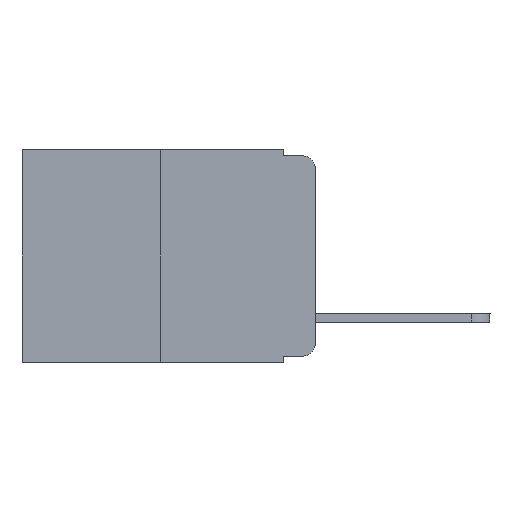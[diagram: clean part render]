
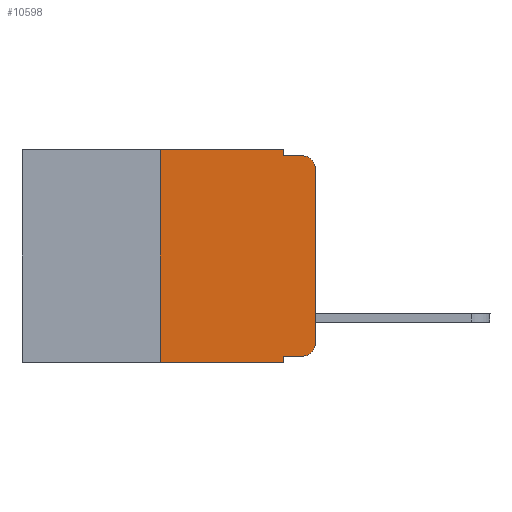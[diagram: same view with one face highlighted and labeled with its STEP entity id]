
A CAD part, left-side view. The second image highlights one B-rep face of the part: STEP entity #10598.
In plain terms, the highlighted planar face has unit normal (-1, 0, 0).
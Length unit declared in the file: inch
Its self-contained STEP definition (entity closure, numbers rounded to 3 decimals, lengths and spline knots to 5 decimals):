
#159 = CARTESIAN_POINT ( 'NONE',  ( 0., 0., -0.03 ) ) ;
#322 = DIRECTION ( 'NONE',  ( 0., 0., 1. ) ) ;
#790 = CARTESIAN_POINT ( 'NONE',  ( 0., 0.473, -0.343 ) ) ;
#799 = ORIENTED_EDGE ( 'NONE', *, *, #14984, .F. ) ;
#1179 = DIRECTION ( 'NONE',  ( 0., 0., -1. ) ) ;
#1741 = VERTEX_POINT ( 'NONE', #6451 ) ;
#1980 = VERTEX_POINT ( 'NONE', #14665 ) ;
#1996 = LINE ( 'NONE', #13366, #11651 ) ;
#2270 = VERTEX_POINT ( 'NONE', #159 ) ;
#2377 = CARTESIAN_POINT ( 'NONE',  ( 0., 0., -0.313 ) ) ;
#2961 = PLANE ( 'NONE',  #17965 ) ;
#2963 = CIRCLE ( 'NONE', #3658, 0.02 ) ;
#3137 = VECTOR ( 'NONE', #13994, 39.37008 ) ;
#3658 = AXIS2_PLACEMENT_3D ( 'NONE', #4294, #9281, #1179 ) ;
#4294 = CARTESIAN_POINT ( 'NONE',  ( 0., 0.02, -0.313 ) ) ;
#4512 = LINE ( 'NONE', #5972, #3137 ) ;
#4913 = LINE ( 'NONE', #14594, #5388 ) ;
#4922 = AXIS2_PLACEMENT_3D ( 'NONE', #5333, #8553, #7001 ) ;
#4974 = ORIENTED_EDGE ( 'NONE', *, *, #9706, .T. ) ;
#5072 = DIRECTION ( 'NONE',  ( 0., -1., 0. ) ) ;
#5231 = DIRECTION ( 'NONE',  ( 0., 0., -1. ) ) ;
#5333 = CARTESIAN_POINT ( 'NONE',  ( 0., 0.02, -0.03 ) ) ;
#5388 = VECTOR ( 'NONE', #322, 39.37008 ) ;
#5605 = VECTOR ( 'NONE', #5231, 39.37008 ) ;
#5791 = DIRECTION ( 'NONE',  ( 1., 0., 0. ) ) ;
#5972 = CARTESIAN_POINT ( 'NONE',  ( 0., 0.051, -0.01 ) ) ;
#6451 = CARTESIAN_POINT ( 'NONE',  ( 0., 0.051, -0.01 ) ) ;
#6452 = VECTOR ( 'NONE', #17511, 39.37008 ) ;
#6668 = EDGE_CURVE ( 'NONE', #1741, #20434, #4512, .T. ) ;
#6861 = ORIENTED_EDGE ( 'NONE', *, *, #16274, .F. ) ;
#6928 = ORIENTED_EDGE ( 'NONE', *, *, #17504, .T. ) ;
#7001 = DIRECTION ( 'NONE',  ( 0., 0., -1. ) ) ;
#8553 = DIRECTION ( 'NONE',  ( -1., 0., 0. ) ) ;
#8707 = CARTESIAN_POINT ( 'NONE',  ( 0., 0.02, -0.333 ) ) ;
#8718 = ORIENTED_EDGE ( 'NONE', *, *, #6668, .F. ) ;
#8801 = DIRECTION ( 'NONE',  ( 0., -1., 0. ) ) ;
#9027 = DIRECTION ( 'NONE',  ( 0., 0., 1. ) ) ;
#9128 = LINE ( 'NONE', #12585, #12648 ) ;
#9272 = CARTESIAN_POINT ( 'NONE',  ( 0., 0.02, -0.01 ) ) ;
#9281 = DIRECTION ( 'NONE',  ( -1., 0., 0. ) ) ;
#9706 = EDGE_CURVE ( 'NONE', #2270, #20434, #16221, .T. ) ;
#9904 = CARTESIAN_POINT ( 'NONE',  ( 0., 0.051, 0. ) ) ;
#10477 = VERTEX_POINT ( 'NONE', #11844 ) ;
#10568 = DIRECTION ( 'NONE',  ( 0., 0., -1. ) ) ;
#10598 = ADVANCED_FACE ( 'NONE', ( #20229 ), #2961, .F. ) ;
#11294 = VERTEX_POINT ( 'NONE', #2377 ) ;
#11359 = CARTESIAN_POINT ( 'NONE',  ( 0., 0.051, -0.343 ) ) ;
#11387 = EDGE_CURVE ( 'NONE', #10477, #1980, #9128, .T. ) ;
#11530 = EDGE_CURVE ( 'NONE', #1980, #18431, #15798, .T. ) ;
#11651 = VECTOR ( 'NONE', #16272, 39.37008 ) ;
#11844 = CARTESIAN_POINT ( 'NONE',  ( 0., 0.25, -0.343 ) ) ;
#12585 = CARTESIAN_POINT ( 'NONE',  ( 0., 0.25, 0. ) ) ;
#12648 = VECTOR ( 'NONE', #9027, 39.37008 ) ;
#12900 = EDGE_CURVE ( 'NONE', #10477, #17775, #17859, .T. ) ;
#13278 = ORIENTED_EDGE ( 'NONE', *, *, #20552, .T. ) ;
#13366 = CARTESIAN_POINT ( 'NONE',  ( 0., 0.051, -0.333 ) ) ;
#13807 = CARTESIAN_POINT ( 'NONE',  ( 0., 0.473, 0. ) ) ;
#13877 = ORIENTED_EDGE ( 'NONE', *, *, #11387, .F. ) ;
#13994 = DIRECTION ( 'NONE',  ( 0., -1., 0. ) ) ;
#14226 = VERTEX_POINT ( 'NONE', #8707 ) ;
#14594 = CARTESIAN_POINT ( 'NONE',  ( 0., 0., 0. ) ) ;
#14665 = CARTESIAN_POINT ( 'NONE',  ( 0., 0.25, 0. ) ) ;
#14984 = EDGE_CURVE ( 'NONE', #18431, #1741, #18835, .T. ) ;
#15015 = CARTESIAN_POINT ( 'NONE',  ( 0., 0.051, -0.333 ) ) ;
#15157 = VERTEX_POINT ( 'NONE', #15015 ) ;
#15343 = VECTOR ( 'NONE', #5072, 39.37008 ) ;
#15798 = LINE ( 'NONE', #17555, #15343 ) ;
#15803 = ORIENTED_EDGE ( 'NONE', *, *, #17177, .T. ) ;
#16221 = CIRCLE ( 'NONE', #4922, 0.02 ) ;
#16272 = DIRECTION ( 'NONE',  ( 0., -1., 0. ) ) ;
#16274 = EDGE_CURVE ( 'NONE', #15157, #17775, #17817, .T. ) ;
#16517 = ORIENTED_EDGE ( 'NONE', *, *, #12900, .T. ) ;
#17177 = EDGE_CURVE ( 'NONE', #14226, #11294, #2963, .T. ) ;
#17504 = EDGE_CURVE ( 'NONE', #15157, #14226, #1996, .T. ) ;
#17511 = DIRECTION ( 'NONE',  ( 0., 0., -1. ) ) ;
#17555 = CARTESIAN_POINT ( 'NONE',  ( 0., 0.473, 0. ) ) ;
#17775 = VERTEX_POINT ( 'NONE', #11359 ) ;
#17817 = LINE ( 'NONE', #9904, #5605 ) ;
#17859 = LINE ( 'NONE', #790, #20316 ) ;
#17965 = AXIS2_PLACEMENT_3D ( 'NONE', #13807, #5791, #10568 ) ;
#18431 = VERTEX_POINT ( 'NONE', #19931 ) ;
#18835 = LINE ( 'NONE', #20411, #6452 ) ;
#19176 = ORIENTED_EDGE ( 'NONE', *, *, #11530, .F. ) ;
#19726 = EDGE_LOOP ( 'NONE', ( #13278, #4974, #8718, #799, #19176, #13877, #16517, #6861, #6928, #15803 ) ) ;
#19931 = CARTESIAN_POINT ( 'NONE',  ( 0., 0.051, 0. ) ) ;
#20229 = FACE_OUTER_BOUND ( 'NONE', #19726, .T. ) ;
#20316 = VECTOR ( 'NONE', #8801, 39.37008 ) ;
#20411 = CARTESIAN_POINT ( 'NONE',  ( 0., 0.051, 0. ) ) ;
#20434 = VERTEX_POINT ( 'NONE', #9272 ) ;
#20552 = EDGE_CURVE ( 'NONE', #11294, #2270, #4913, .T. ) ;
